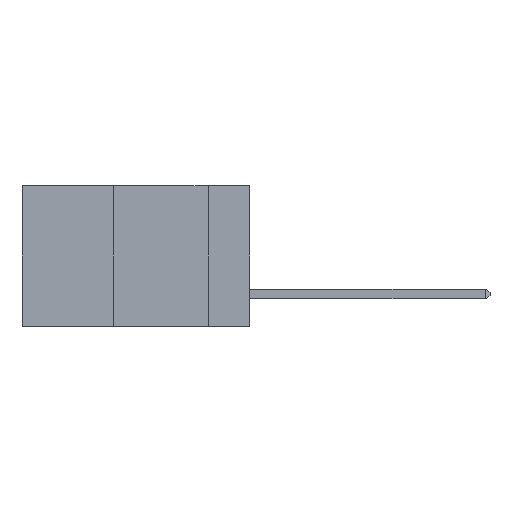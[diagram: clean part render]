
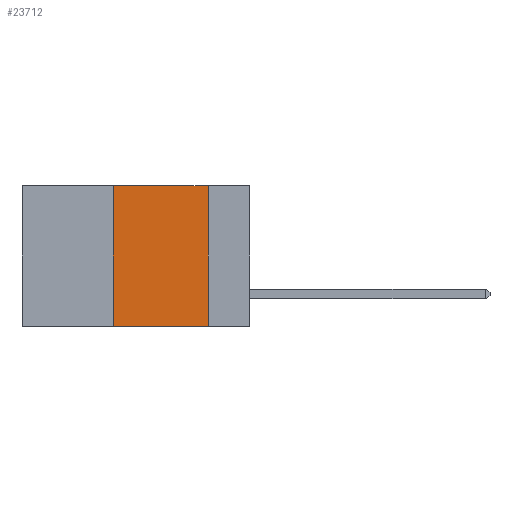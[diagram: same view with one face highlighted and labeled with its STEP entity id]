
A CAD part, left-side view. The second image highlights one B-rep face of the part: STEP entity #23712.
In plain terms, the highlighted planar face has unit normal (-1, 0, 0).
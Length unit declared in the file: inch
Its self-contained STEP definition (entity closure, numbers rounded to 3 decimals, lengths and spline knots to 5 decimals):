
#520 = CARTESIAN_POINT ( 'NONE',  ( 0., 0.11, 0. ) ) ;
#2883 = DIRECTION ( 'NONE',  ( 0., -1., 0. ) ) ;
#2896 = CARTESIAN_POINT ( 'NONE',  ( 0., 0.36, 0. ) ) ;
#3571 = ORIENTED_EDGE ( 'NONE', *, *, #5108, .T. ) ;
#4576 = EDGE_LOOP ( 'NONE', ( #13351, #23055, #9272, #3571 ) ) ;
#5108 = EDGE_CURVE ( 'NONE', #23466, #27257, #34825, .T. ) ;
#5116 = VERTEX_POINT ( 'NONE', #19890 ) ;
#5709 = DIRECTION ( 'NONE',  ( 0., 0., 1. ) ) ;
#6748 = LINE ( 'NONE', #30645, #35523 ) ;
#9272 = ORIENTED_EDGE ( 'NONE', *, *, #28127, .F. ) ;
#10162 = CARTESIAN_POINT ( 'NONE',  ( 0., 0.6, 0. ) ) ;
#11480 = DIRECTION ( 'NONE',  ( 0., -1., 0. ) ) ;
#12811 = EDGE_CURVE ( 'NONE', #5116, #30952, #6748, .T. ) ;
#12960 = DIRECTION ( 'NONE',  ( 0., 0., -1. ) ) ;
#13351 = ORIENTED_EDGE ( 'NONE', *, *, #20427, .F. ) ;
#18253 = VECTOR ( 'NONE', #11480, 39.37008 ) ;
#19890 = CARTESIAN_POINT ( 'NONE',  ( 0., 0.36, 0. ) ) ;
#20002 = DIRECTION ( 'NONE',  ( 0., 0., -1. ) ) ;
#20427 = EDGE_CURVE ( 'NONE', #30952, #27257, #32503, .T. ) ;
#21827 = FACE_OUTER_BOUND ( 'NONE', #4576, .T. ) ;
#23055 = ORIENTED_EDGE ( 'NONE', *, *, #12811, .F. ) ;
#23466 = VERTEX_POINT ( 'NONE', #24076 ) ;
#23712 = ADVANCED_FACE ( 'NONE', ( #21827 ), #26834, .F. ) ;
#24076 = CARTESIAN_POINT ( 'NONE',  ( 0., 0.36, -0.37 ) ) ;
#25098 = VECTOR ( 'NONE', #20002, 39.37008 ) ;
#25357 = CARTESIAN_POINT ( 'NONE',  ( 0., 0.6, -0.37 ) ) ;
#25987 = LINE ( 'NONE', #2896, #26881 ) ;
#26834 = PLANE ( 'NONE',  #32549 ) ;
#26881 = VECTOR ( 'NONE', #5709, 39.37008 ) ;
#26955 = CARTESIAN_POINT ( 'NONE',  ( 0., 0.11, -0.37 ) ) ;
#27257 = VERTEX_POINT ( 'NONE', #26955 ) ;
#28127 = EDGE_CURVE ( 'NONE', #23466, #5116, #25987, .T. ) ;
#29627 = DIRECTION ( 'NONE',  ( 1., 0., 0. ) ) ;
#30645 = CARTESIAN_POINT ( 'NONE',  ( 0., 0.6, 0. ) ) ;
#30952 = VERTEX_POINT ( 'NONE', #32357 ) ;
#32357 = CARTESIAN_POINT ( 'NONE',  ( 0., 0.11, 0. ) ) ;
#32503 = LINE ( 'NONE', #520, #25098 ) ;
#32549 = AXIS2_PLACEMENT_3D ( 'NONE', #10162, #29627, #12960 ) ;
#34825 = LINE ( 'NONE', #25357, #18253 ) ;
#35523 = VECTOR ( 'NONE', #2883, 39.37008 ) ;
